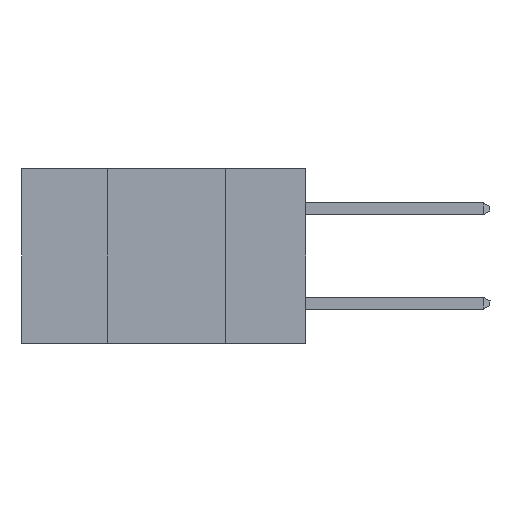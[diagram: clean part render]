
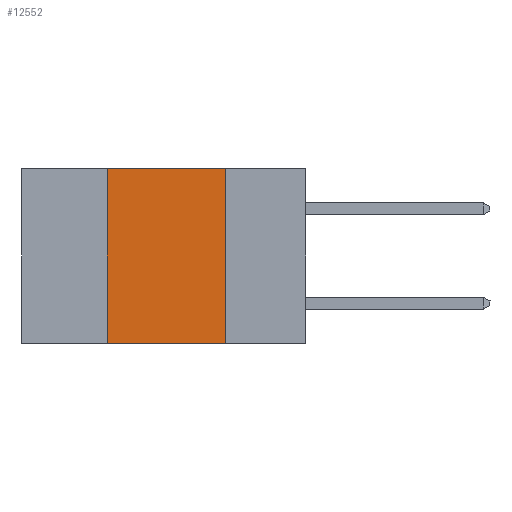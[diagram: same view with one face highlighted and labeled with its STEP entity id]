
A CAD part, left-side view. The second image highlights one B-rep face of the part: STEP entity #12552.
In plain terms, the highlighted planar face has unit normal (-1, 0, 0).
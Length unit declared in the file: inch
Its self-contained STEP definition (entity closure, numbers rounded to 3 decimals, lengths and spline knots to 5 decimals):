
#81 = DIRECTION ( 'NONE',  ( 0., 0., -1. ) ) ;
#99 = CARTESIAN_POINT ( 'NONE',  ( 0., 0.17, -0.37 ) ) ;
#383 = LINE ( 'NONE', #9784, #9904 ) ;
#774 = LINE ( 'NONE', #7814, #7329 ) ;
#849 = DIRECTION ( 'NONE',  ( 0., 0., 1. ) ) ;
#914 = CARTESIAN_POINT ( 'NONE',  ( 0., 0.42, -0.37 ) ) ;
#1212 = CARTESIAN_POINT ( 'NONE',  ( 0., 0.42, 0. ) ) ;
#1248 = EDGE_LOOP ( 'NONE', ( #6093, #4840, #8673, #13155 ) ) ;
#3935 = VERTEX_POINT ( 'NONE', #14248 ) ;
#4078 = VECTOR ( 'NONE', #81, 39.37008 ) ;
#4660 = VERTEX_POINT ( 'NONE', #15802 ) ;
#4840 = ORIENTED_EDGE ( 'NONE', *, *, #14012, .F. ) ;
#4902 = LINE ( 'NONE', #99, #4078 ) ;
#4958 = VECTOR ( 'NONE', #849, 39.37008 ) ;
#5345 = LINE ( 'NONE', #914, #4958 ) ;
#6093 = ORIENTED_EDGE ( 'NONE', *, *, #11773, .F. ) ;
#6880 = EDGE_CURVE ( 'NONE', #15389, #3935, #383, .T. ) ;
#7329 = VECTOR ( 'NONE', #10437, 39.37008 ) ;
#7814 = CARTESIAN_POINT ( 'NONE',  ( 0., 0.6, 0. ) ) ;
#8381 = AXIS2_PLACEMENT_3D ( 'NONE', #8930, #8872, #8854 ) ;
#8673 = ORIENTED_EDGE ( 'NONE', *, *, #9153, .F. ) ;
#8854 = DIRECTION ( 'NONE',  ( 0., 0., -1. ) ) ;
#8872 = DIRECTION ( 'NONE',  ( 1., 0., 0. ) ) ;
#8896 = PLANE ( 'NONE',  #8381 ) ;
#8930 = CARTESIAN_POINT ( 'NONE',  ( 0., 0.6, 0. ) ) ;
#9153 = EDGE_CURVE ( 'NONE', #15389, #13926, #5345, .T. ) ;
#9368 = CARTESIAN_POINT ( 'NONE',  ( 0., 0.42, -0.37 ) ) ;
#9784 = CARTESIAN_POINT ( 'NONE',  ( 0., 0.6, -0.37 ) ) ;
#9904 = VECTOR ( 'NONE', #10085, 39.37008 ) ;
#10085 = DIRECTION ( 'NONE',  ( 0., -1., 0. ) ) ;
#10437 = DIRECTION ( 'NONE',  ( 0., -1., 0. ) ) ;
#11773 = EDGE_CURVE ( 'NONE', #4660, #3935, #4902, .T. ) ;
#12535 = FACE_OUTER_BOUND ( 'NONE', #1248, .T. ) ;
#12552 = ADVANCED_FACE ( 'NONE', ( #12535 ), #8896, .F. ) ;
#13155 = ORIENTED_EDGE ( 'NONE', *, *, #6880, .T. ) ;
#13926 = VERTEX_POINT ( 'NONE', #1212 ) ;
#14012 = EDGE_CURVE ( 'NONE', #13926, #4660, #774, .T. ) ;
#14248 = CARTESIAN_POINT ( 'NONE',  ( 0., 0.17, -0.37 ) ) ;
#15389 = VERTEX_POINT ( 'NONE', #9368 ) ;
#15802 = CARTESIAN_POINT ( 'NONE',  ( 0., 0.17, 0. ) ) ;
